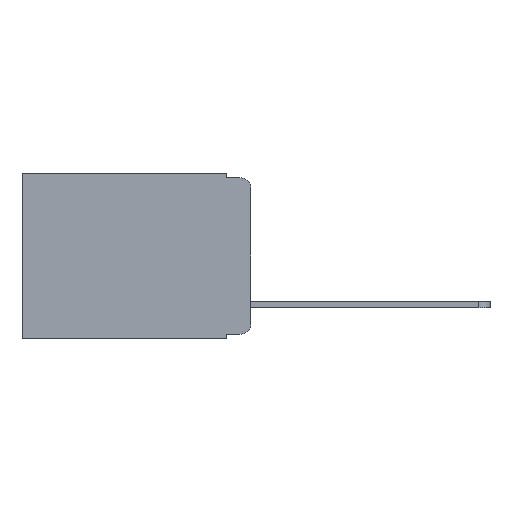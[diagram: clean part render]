
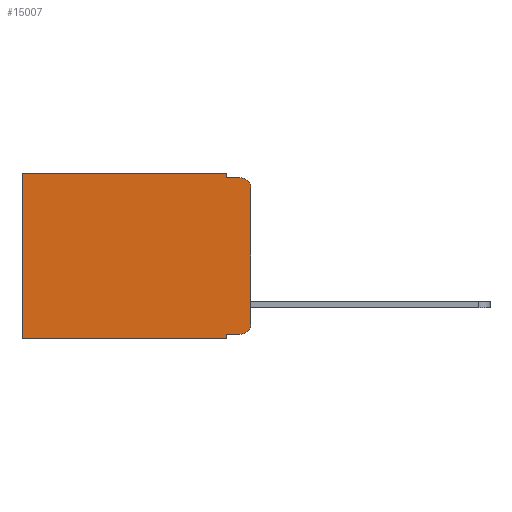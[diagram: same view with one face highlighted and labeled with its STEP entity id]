
A CAD part, left-side view. The second image highlights one B-rep face of the part: STEP entity #15007.
In plain terms, the highlighted planar face has unit normal (-1, 0, 0).
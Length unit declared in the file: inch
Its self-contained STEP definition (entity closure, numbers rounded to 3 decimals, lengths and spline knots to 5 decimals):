
#348 = ORIENTED_EDGE ( 'NONE', *, *, #23405, .T. ) ;
#401 = ORIENTED_EDGE ( 'NONE', *, *, #19111, .F. ) ;
#1033 = CARTESIAN_POINT ( 'NONE',  ( 0.298, 0.051, -0.01 ) ) ;
#2054 = CARTESIAN_POINT ( 'NONE',  ( 0.298, 0.473, 0. ) ) ;
#2058 = DIRECTION ( 'NONE',  ( 0., 1., 0. ) ) ;
#2585 = ORIENTED_EDGE ( 'NONE', *, *, #10299, .F. ) ;
#2647 = DIRECTION ( 'NONE',  ( 0., 0., -1. ) ) ;
#2650 = ORIENTED_EDGE ( 'NONE', *, *, #21724, .F. ) ;
#2658 = PLANE ( 'NONE',  #20186 ) ;
#3045 = LINE ( 'NONE', #9699, #12283 ) ;
#3206 = DIRECTION ( 'NONE',  ( 0., -1., 0. ) ) ;
#4116 = VERTEX_POINT ( 'NONE', #2054 ) ;
#4227 = ORIENTED_EDGE ( 'NONE', *, *, #16347, .T. ) ;
#4357 = AXIS2_PLACEMENT_3D ( 'NONE', #19928, #4711, #2647 ) ;
#4511 = AXIS2_PLACEMENT_3D ( 'NONE', #8846, #7083, #20298 ) ;
#4711 = DIRECTION ( 'NONE',  ( -1., 0., 0. ) ) ;
#5250 = LINE ( 'NONE', #1033, #22857 ) ;
#5821 = CIRCLE ( 'NONE', #4511, 0.02 ) ;
#5981 = VECTOR ( 'NONE', #23453, 39.37008 ) ;
#6058 = CARTESIAN_POINT ( 'NONE',  ( 0.298, 0., 0. ) ) ;
#6355 = CARTESIAN_POINT ( 'NONE',  ( 0.298, 0.051, -0.333 ) ) ;
#6456 = CARTESIAN_POINT ( 'NONE',  ( 0.298, 0.02, -0.333 ) ) ;
#6719 = VERTEX_POINT ( 'NONE', #17734 ) ;
#6874 = VERTEX_POINT ( 'NONE', #10263 ) ;
#7083 = DIRECTION ( 'NONE',  ( -1., 0., 0. ) ) ;
#7402 = DIRECTION ( 'NONE',  ( 0., 1., 0. ) ) ;
#7451 = EDGE_CURVE ( 'NONE', #18112, #6719, #19789, .T. ) ;
#7845 = EDGE_CURVE ( 'NONE', #8322, #23361, #3045, .T. ) ;
#7999 = CARTESIAN_POINT ( 'NONE',  ( 0.298, 0.051, -0.01 ) ) ;
#8322 = VERTEX_POINT ( 'NONE', #17309 ) ;
#8846 = CARTESIAN_POINT ( 'NONE',  ( 0.298, 0.02, -0.03 ) ) ;
#9661 = ORIENTED_EDGE ( 'NONE', *, *, #7845, .F. ) ;
#9699 = CARTESIAN_POINT ( 'NONE',  ( 0.298, 0., -0.343 ) ) ;
#9859 = CARTESIAN_POINT ( 'NONE',  ( 0.298, 0.473, -0.343 ) ) ;
#10229 = CARTESIAN_POINT ( 'NONE',  ( 0.298, 0.051, -0.333 ) ) ;
#10263 = CARTESIAN_POINT ( 'NONE',  ( 0.298, 0.02, -0.01 ) ) ;
#10299 = EDGE_CURVE ( 'NONE', #21680, #23482, #10346, .T. ) ;
#10301 = CARTESIAN_POINT ( 'NONE',  ( 0.298, 0.473, 0. ) ) ;
#10346 = LINE ( 'NONE', #11972, #19925 ) ;
#10403 = CARTESIAN_POINT ( 'NONE',  ( 0.298, 0., 0. ) ) ;
#10578 = VERTEX_POINT ( 'NONE', #14736 ) ;
#11503 = CARTESIAN_POINT ( 'NONE',  ( 0.298, 0.051, 0. ) ) ;
#11907 = FACE_OUTER_BOUND ( 'NONE', #18339, .T. ) ;
#11972 = CARTESIAN_POINT ( 'NONE',  ( 0.298, 0.051, 0. ) ) ;
#12126 = DIRECTION ( 'NONE',  ( 0., 0., -1. ) ) ;
#12283 = VECTOR ( 'NONE', #2058, 39.37008 ) ;
#12359 = VECTOR ( 'NONE', #7402, 39.37008 ) ;
#12415 = EDGE_CURVE ( 'NONE', #21680, #4116, #19825, .T. ) ;
#12423 = DIRECTION ( 'NONE',  ( 0., 0., -1. ) ) ;
#12497 = DIRECTION ( 'NONE',  ( 0., 0., -1. ) ) ;
#14642 = LINE ( 'NONE', #6355, #22088 ) ;
#14736 = CARTESIAN_POINT ( 'NONE',  ( 0.298, 0., -0.03 ) ) ;
#14975 = VECTOR ( 'NONE', #12497, 39.37008 ) ;
#15007 = ADVANCED_FACE ( 'NONE', ( #11907 ), #2658, .F. ) ;
#15215 = DIRECTION ( 'NONE',  ( 0., 0., -1. ) ) ;
#15919 = CARTESIAN_POINT ( 'NONE',  ( 0.298, 0.051, 0. ) ) ;
#16347 = EDGE_CURVE ( 'NONE', #10578, #6874, #5821, .T. ) ;
#16383 = ORIENTED_EDGE ( 'NONE', *, *, #7451, .T. ) ;
#16762 = LINE ( 'NONE', #10301, #14975 ) ;
#17309 = CARTESIAN_POINT ( 'NONE',  ( 0.298, 0.051, -0.343 ) ) ;
#17432 = ORIENTED_EDGE ( 'NONE', *, *, #22747, .F. ) ;
#17443 = ORIENTED_EDGE ( 'NONE', *, *, #12415, .T. ) ;
#17658 = DIRECTION ( 'NONE',  ( 0., -1., 0. ) ) ;
#17734 = CARTESIAN_POINT ( 'NONE',  ( 0.298, 0., -0.313 ) ) ;
#17950 = DIRECTION ( 'NONE',  ( 1., 0., 0. ) ) ;
#18112 = VERTEX_POINT ( 'NONE', #6456 ) ;
#18339 = EDGE_LOOP ( 'NONE', ( #17432, #4227, #2650, #2585, #17443, #22616, #9661, #401, #348, #16383 ) ) ;
#19111 = EDGE_CURVE ( 'NONE', #22917, #8322, #23304, .T. ) ;
#19789 = CIRCLE ( 'NONE', #4357, 0.02 ) ;
#19825 = LINE ( 'NONE', #22207, #12359 ) ;
#19925 = VECTOR ( 'NONE', #12126, 39.37008 ) ;
#19928 = CARTESIAN_POINT ( 'NONE',  ( 0.298, 0.02, -0.313 ) ) ;
#20186 = AXIS2_PLACEMENT_3D ( 'NONE', #10403, #17950, #12423 ) ;
#20298 = DIRECTION ( 'NONE',  ( 0., 0., -1. ) ) ;
#21228 = LINE ( 'NONE', #6058, #5981 ) ;
#21680 = VERTEX_POINT ( 'NONE', #15919 ) ;
#21724 = EDGE_CURVE ( 'NONE', #23482, #6874, #5250, .T. ) ;
#22088 = VECTOR ( 'NONE', #17658, 39.37008 ) ;
#22207 = CARTESIAN_POINT ( 'NONE',  ( 0.298, 0., 0. ) ) ;
#22616 = ORIENTED_EDGE ( 'NONE', *, *, #22915, .T. ) ;
#22747 = EDGE_CURVE ( 'NONE', #10578, #6719, #21228, .T. ) ;
#22857 = VECTOR ( 'NONE', #3206, 39.37008 ) ;
#22915 = EDGE_CURVE ( 'NONE', #4116, #23361, #16762, .T. ) ;
#22917 = VERTEX_POINT ( 'NONE', #10229 ) ;
#23304 = LINE ( 'NONE', #11503, #23602 ) ;
#23361 = VERTEX_POINT ( 'NONE', #9859 ) ;
#23405 = EDGE_CURVE ( 'NONE', #22917, #18112, #14642, .T. ) ;
#23453 = DIRECTION ( 'NONE',  ( 0., 0., -1. ) ) ;
#23482 = VERTEX_POINT ( 'NONE', #7999 ) ;
#23602 = VECTOR ( 'NONE', #15215, 39.37008 ) ;
